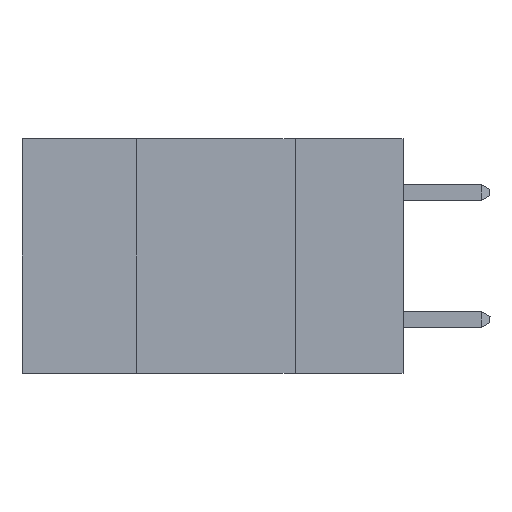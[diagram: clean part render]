
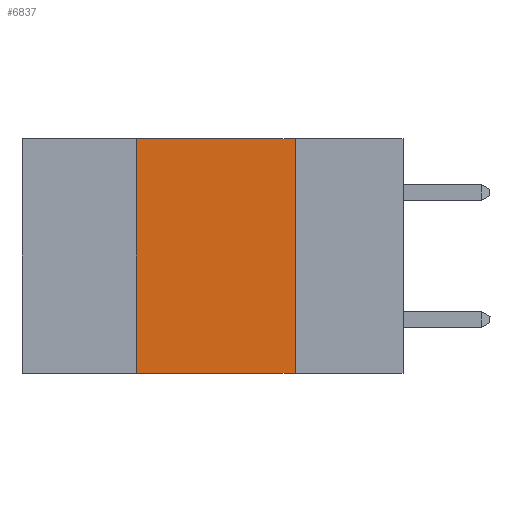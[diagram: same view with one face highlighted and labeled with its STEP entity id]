
A CAD part, left-side view. The second image highlights one B-rep face of the part: STEP entity #6837.
In plain terms, the highlighted planar face has unit normal (-1, 0, 0).
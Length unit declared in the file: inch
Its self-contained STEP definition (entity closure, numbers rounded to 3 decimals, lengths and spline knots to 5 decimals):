
#571 = ORIENTED_EDGE ( 'NONE', *, *, #14932, .F. ) ;
#936 = EDGE_CURVE ( 'NONE', #5259, #1519, #4939, .T. ) ;
#1082 = CARTESIAN_POINT ( 'NONE',  ( 0., 0.17, -0.37 ) ) ;
#1519 = VERTEX_POINT ( 'NONE', #12921 ) ;
#2447 = VECTOR ( 'NONE', #11205, 39.37008 ) ;
#2475 = CARTESIAN_POINT ( 'NONE',  ( 0., 0.42, 0. ) ) ;
#2794 = LINE ( 'NONE', #2475, #2447 ) ;
#3281 = EDGE_CURVE ( 'NONE', #1519, #8722, #8581, .T. ) ;
#3913 = VERTEX_POINT ( 'NONE', #7980 ) ;
#4435 = CARTESIAN_POINT ( 'NONE',  ( 0., 0.6, -0.37 ) ) ;
#4939 = LINE ( 'NONE', #12533, #13715 ) ;
#5259 = VERTEX_POINT ( 'NONE', #11714 ) ;
#5906 = CARTESIAN_POINT ( 'NONE',  ( 0., 0.6, 0. ) ) ;
#6837 = ADVANCED_FACE ( 'NONE', ( #8327 ), #12055, .F. ) ;
#7387 = ORIENTED_EDGE ( 'NONE', *, *, #12958, .T. ) ;
#7980 = CARTESIAN_POINT ( 'NONE',  ( 0., 0.42, -0.37 ) ) ;
#8327 = FACE_OUTER_BOUND ( 'NONE', #8875, .T. ) ;
#8546 = ORIENTED_EDGE ( 'NONE', *, *, #936, .F. ) ;
#8581 = LINE ( 'NONE', #14825, #12352 ) ;
#8663 = DIRECTION ( 'NONE',  ( 0., 0., -1. ) ) ;
#8722 = VERTEX_POINT ( 'NONE', #1082 ) ;
#8875 = EDGE_LOOP ( 'NONE', ( #14431, #8546, #571, #7387 ) ) ;
#9637 = DIRECTION ( 'NONE',  ( 0., 0., -1. ) ) ;
#11205 = DIRECTION ( 'NONE',  ( 0., 0., 1. ) ) ;
#11714 = CARTESIAN_POINT ( 'NONE',  ( 0., 0.42, 0. ) ) ;
#11889 = LINE ( 'NONE', #4435, #13524 ) ;
#12055 = PLANE ( 'NONE',  #12393 ) ;
#12352 = VECTOR ( 'NONE', #8663, 39.37008 ) ;
#12393 = AXIS2_PLACEMENT_3D ( 'NONE', #5906, #15782, #9637 ) ;
#12533 = CARTESIAN_POINT ( 'NONE',  ( 0., 0.6, 0. ) ) ;
#12921 = CARTESIAN_POINT ( 'NONE',  ( 0., 0.17, 0. ) ) ;
#12958 = EDGE_CURVE ( 'NONE', #3913, #8722, #11889, .T. ) ;
#13524 = VECTOR ( 'NONE', #14153, 39.37008 ) ;
#13715 = VECTOR ( 'NONE', #14828, 39.37008 ) ;
#14153 = DIRECTION ( 'NONE',  ( 0., -1., 0. ) ) ;
#14431 = ORIENTED_EDGE ( 'NONE', *, *, #3281, .F. ) ;
#14825 = CARTESIAN_POINT ( 'NONE',  ( 0., 0.17, 0. ) ) ;
#14828 = DIRECTION ( 'NONE',  ( 0., -1., 0. ) ) ;
#14932 = EDGE_CURVE ( 'NONE', #3913, #5259, #2794, .T. ) ;
#15782 = DIRECTION ( 'NONE',  ( 1., 0., 0. ) ) ;
